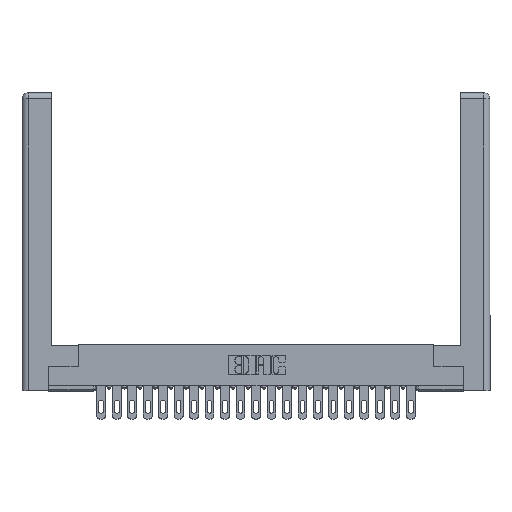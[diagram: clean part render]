
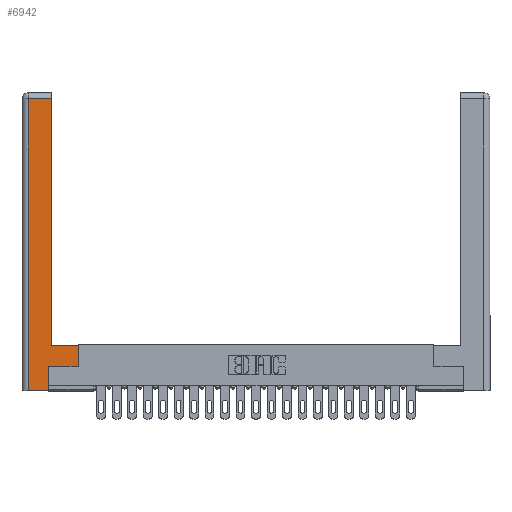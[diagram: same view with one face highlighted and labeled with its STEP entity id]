
A CAD part, top view. The second image highlights one B-rep face of the part: STEP entity #6942.
In plain terms, the highlighted planar face has unit normal (0, 0, 1).
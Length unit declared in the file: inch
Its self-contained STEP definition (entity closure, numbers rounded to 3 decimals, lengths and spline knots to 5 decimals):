
#364 = LINE ( 'NONE', #9605, #2668 ) ;
#482 = EDGE_CURVE ( 'NONE', #12586, #13652, #19437, .T. ) ;
#597 = EDGE_CURVE ( 'NONE', #11160, #18424, #2105, .T. ) ;
#701 = VERTEX_POINT ( 'NONE', #1621 ) ;
#1364 = FACE_OUTER_BOUND ( 'NONE', #21495, .T. ) ;
#1621 = CARTESIAN_POINT ( 'NONE',  ( 0.0615, 2.94, 0. ) ) ;
#2105 = LINE ( 'NONE', #17829, #21413 ) ;
#2668 = VECTOR ( 'NONE', #13682, 39.37008 ) ;
#3836 = DIRECTION ( 'NONE',  ( 0., 0., -1. ) ) ;
#4101 = ORIENTED_EDGE ( 'NONE', *, *, #7036, .T. ) ;
#4182 = CARTESIAN_POINT ( 'NONE',  ( 0.265, 0.245, 0. ) ) ;
#4646 = CARTESIAN_POINT ( 'NONE',  ( 0.565, 0.45, 0. ) ) ;
#4756 = LINE ( 'NONE', #15027, #23786 ) ;
#4866 = VECTOR ( 'NONE', #9769, 39.37008 ) ;
#5932 = ORIENTED_EDGE ( 'NONE', *, *, #18407, .T. ) ;
#6077 = CARTESIAN_POINT ( 'NONE',  ( 0.265, 0.245, 0. ) ) ;
#6549 = DIRECTION ( 'NONE',  ( 1., 0., 0. ) ) ;
#6942 = ADVANCED_FACE ( 'NONE', ( #1364 ), #18524, .F. ) ;
#7036 = EDGE_CURVE ( 'NONE', #13652, #11160, #8869, .T. ) ;
#7790 = VERTEX_POINT ( 'NONE', #11955 ) ;
#8869 = LINE ( 'NONE', #6077, #15190 ) ;
#9176 = DIRECTION ( 'NONE',  ( -1., 0., 0. ) ) ;
#9605 = CARTESIAN_POINT ( 'NONE',  ( 0.0615, 0., 0. ) ) ;
#9769 = DIRECTION ( 'NONE',  ( 0., 1., 0. ) ) ;
#10384 = DIRECTION ( 'NONE',  ( 0., 1., 0. ) ) ;
#10460 = VECTOR ( 'NONE', #9176, 39.37008 ) ;
#11160 = VERTEX_POINT ( 'NONE', #4182 ) ;
#11467 = ORIENTED_EDGE ( 'NONE', *, *, #23543, .T. ) ;
#11470 = CARTESIAN_POINT ( 'NONE',  ( 0.565, 0.45, 0. ) ) ;
#11628 = VECTOR ( 'NONE', #6549, 39.37008 ) ;
#11871 = ORIENTED_EDGE ( 'NONE', *, *, #597, .T. ) ;
#11955 = CARTESIAN_POINT ( 'NONE',  ( 0.295, 0.45, 0. ) ) ;
#12151 = CARTESIAN_POINT ( 'NONE',  ( 0.295, 3., 0. ) ) ;
#12188 = LINE ( 'NONE', #16080, #10460 ) ;
#12586 = VERTEX_POINT ( 'NONE', #18877 ) ;
#12674 = AXIS2_PLACEMENT_3D ( 'NONE', #14876, #3836, #22283 ) ;
#12696 = EDGE_CURVE ( 'NONE', #701, #12586, #364, .T. ) ;
#12973 = EDGE_CURVE ( 'NONE', #23220, #701, #12188, .T. ) ;
#13437 = CARTESIAN_POINT ( 'NONE',  ( 0.295, 2.94, 0. ) ) ;
#13652 = VERTEX_POINT ( 'NONE', #18345 ) ;
#13682 = DIRECTION ( 'NONE',  ( 0., -1., 0. ) ) ;
#14118 = DIRECTION ( 'NONE',  ( 1., 0., 0. ) ) ;
#14589 = ORIENTED_EDGE ( 'NONE', *, *, #15273, .T. ) ;
#14876 = CARTESIAN_POINT ( 'NONE',  ( 0., 0., 0. ) ) ;
#15027 = CARTESIAN_POINT ( 'NONE',  ( 0.295, 0.45, 0. ) ) ;
#15062 = ORIENTED_EDGE ( 'NONE', *, *, #12973, .T. ) ;
#15098 = LINE ( 'NONE', #12151, #18887 ) ;
#15190 = VECTOR ( 'NONE', #17223, 39.37008 ) ;
#15273 = EDGE_CURVE ( 'NONE', #23357, #7790, #4756, .T. ) ;
#16080 = CARTESIAN_POINT ( 'NONE',  ( 0.0615, 2.94, 0. ) ) ;
#16858 = ORIENTED_EDGE ( 'NONE', *, *, #482, .T. ) ;
#17223 = DIRECTION ( 'NONE',  ( 0., 1., 0. ) ) ;
#17829 = CARTESIAN_POINT ( 'NONE',  ( 0.565, 0.245, 0. ) ) ;
#18345 = CARTESIAN_POINT ( 'NONE',  ( 0.265, 0., 0. ) ) ;
#18407 = EDGE_CURVE ( 'NONE', #18424, #23357, #20194, .T. ) ;
#18424 = VERTEX_POINT ( 'NONE', #19047 ) ;
#18524 = PLANE ( 'NONE',  #12674 ) ;
#18738 = ORIENTED_EDGE ( 'NONE', *, *, #12696, .T. ) ;
#18877 = CARTESIAN_POINT ( 'NONE',  ( 0.0615, 0., 0. ) ) ;
#18887 = VECTOR ( 'NONE', #10384, 39.37008 ) ;
#19047 = CARTESIAN_POINT ( 'NONE',  ( 0.565, 0.245, 0. ) ) ;
#19437 = LINE ( 'NONE', #23053, #11628 ) ;
#20194 = LINE ( 'NONE', #11470, #4866 ) ;
#21413 = VECTOR ( 'NONE', #14118, 39.37008 ) ;
#21495 = EDGE_LOOP ( 'NONE', ( #11467, #15062, #18738, #16858, #4101, #11871, #5932, #14589 ) ) ;
#22283 = DIRECTION ( 'NONE',  ( -1., 0., 0. ) ) ;
#23053 = CARTESIAN_POINT ( 'NONE',  ( 0.265, 0., 0. ) ) ;
#23220 = VERTEX_POINT ( 'NONE', #13437 ) ;
#23357 = VERTEX_POINT ( 'NONE', #4646 ) ;
#23543 = EDGE_CURVE ( 'NONE', #7790, #23220, #15098, .T. ) ;
#23786 = VECTOR ( 'NONE', #23879, 39.37008 ) ;
#23879 = DIRECTION ( 'NONE',  ( -1., 0., 0. ) ) ;
